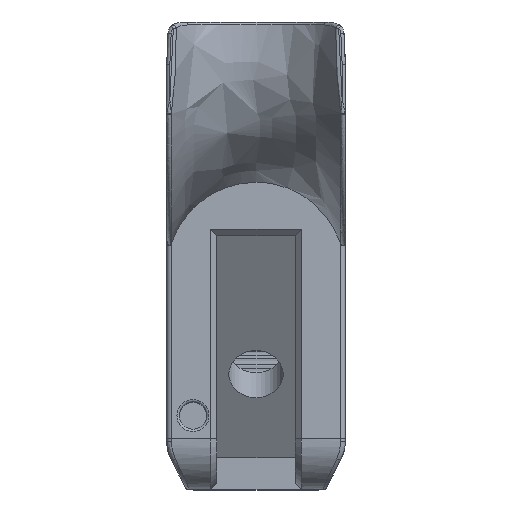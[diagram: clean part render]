
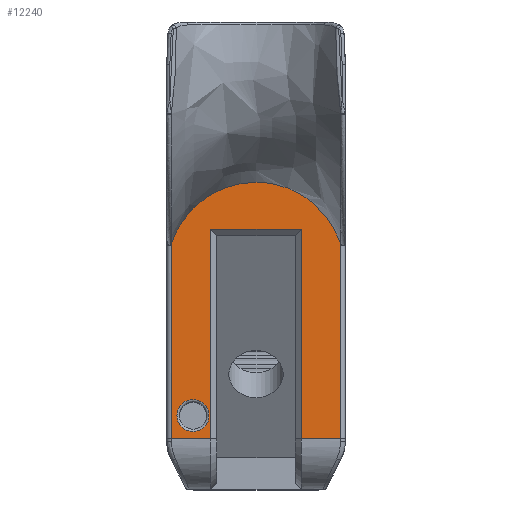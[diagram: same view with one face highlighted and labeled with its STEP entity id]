
A CAD part, top view. The second image highlights one B-rep face of the part: STEP entity #12240.
In plain terms, the highlighted planar face has unit normal (0, 0, 1).
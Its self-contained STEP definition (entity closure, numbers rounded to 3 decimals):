
#243=FACE_BOUND('',#2717,.T.);
#280=PLANE('',#13243);
#452=LINE('',#20827,#1044);
#459=LINE('',#20843,#1051);
#461=LINE('',#21357,#1053);
#485=LINE('',#22272,#1077);
#486=LINE('',#22274,#1078);
#487=LINE('',#22276,#1079);
#488=LINE('',#22278,#1080);
#1044=VECTOR('',#14233,10.);
#1051=VECTOR('',#14250,10.);
#1053=VECTOR('',#14288,10.);
#1077=VECTOR('',#14618,10.);
#1078=VECTOR('',#14619,10.);
#1079=VECTOR('',#14620,10.);
#1080=VECTOR('',#14621,10.);
#1942=FACE_OUTER_BOUND('',#2716,.T.);
#2716=EDGE_LOOP('',(#8739,#8740,#8741,#8742,#8743,#8744,#8745,#8746,#8747));
#2717=EDGE_LOOP('',(#8748));
#3450=B_SPLINE_CURVE_WITH_KNOTS('',3,(#22280,#22281,#22282,#22283,#22284,
#22285,#22286,#22287,#22288,#22289),.UNSPECIFIED.,.F.,.F.,(4,2,2,2,4),(0.313,
0.444,0.89,1.331,1.71),
 .UNSPECIFIED.);
#3451=B_SPLINE_CURVE_WITH_KNOTS('',3,(#22290,#22291,#22292,#22293,#22294,
#22295,#22296,#22297,#22298,#22299,#22300,#22301),.UNSPECIFIED.,.F.,.F.,
(4,2,2,2,2,4),(1.71,1.762,2.19,2.624,
3.022,3.107),.UNSPECIFIED.);
#4323=CIRCLE('',#13095,2.);
#4804=VERTEX_POINT('',#20825);
#4805=VERTEX_POINT('',#20826);
#4809=VERTEX_POINT('',#20842);
#4825=VERTEX_POINT('',#21356);
#4828=VERTEX_POINT('',#21369);
#4902=VERTEX_POINT('',#22271);
#4903=VERTEX_POINT('',#22273);
#4904=VERTEX_POINT('',#22275);
#4905=VERTEX_POINT('',#22277);
#4906=VERTEX_POINT('',#22279);
#6153=EDGE_CURVE('',#4804,#4805,#452,.T.);
#6162=EDGE_CURVE('',#4809,#4805,#459,.T.);
#6193=EDGE_CURVE('',#4809,#4825,#461,.T.);
#6198=EDGE_CURVE('',#4828,#4828,#4323,.T.);
#6338=EDGE_CURVE('',#4902,#4804,#485,.T.);
#6339=EDGE_CURVE('',#4903,#4902,#486,.T.);
#6340=EDGE_CURVE('',#4904,#4903,#487,.T.);
#6341=EDGE_CURVE('',#4905,#4904,#488,.T.);
#6342=EDGE_CURVE('',#4905,#4906,#3450,.T.);
#6343=EDGE_CURVE('',#4906,#4825,#3451,.T.);
#8739=ORIENTED_EDGE('',*,*,#6338,.F.);
#8740=ORIENTED_EDGE('',*,*,#6339,.F.);
#8741=ORIENTED_EDGE('',*,*,#6340,.F.);
#8742=ORIENTED_EDGE('',*,*,#6341,.F.);
#8743=ORIENTED_EDGE('',*,*,#6342,.T.);
#8744=ORIENTED_EDGE('',*,*,#6343,.T.);
#8745=ORIENTED_EDGE('',*,*,#6193,.F.);
#8746=ORIENTED_EDGE('',*,*,#6162,.T.);
#8747=ORIENTED_EDGE('',*,*,#6153,.F.);
#8748=ORIENTED_EDGE('',*,*,#6198,.F.);
#12240=ADVANCED_FACE('',(#1942,#243),#280,.T.);
#13095=AXIS2_PLACEMENT_3D('',#21370,#14298,#14299);
#13243=AXIS2_PLACEMENT_3D('',#22270,#14616,#14617);
#14233=DIRECTION('',(0.,-1.,0.));
#14250=DIRECTION('',(1.,0.,0.));
#14288=DIRECTION('',(0.,1.,0.));
#14298=DIRECTION('center_axis',(0.,0.,
1.));
#14299=DIRECTION('ref_axis',(1.,0.,0.));
#14616=DIRECTION('center_axis',(0.,0.,
1.));
#14617=DIRECTION('ref_axis',(0.,-1.,0.));
#14618=DIRECTION('',(-1.,0.,0.));
#14619=DIRECTION('',(0.,1.,0.));
#14620=DIRECTION('',(-1.,0.,0.));
#14621=DIRECTION('',(0.,-1.,0.));
#20825=CARTESIAN_POINT('',(18.417,-117.318,28.406));
#20826=CARTESIAN_POINT('',(18.417,-143.468,28.406));
#20827=CARTESIAN_POINT('',(18.417,-114.618,28.406));
#20842=CARTESIAN_POINT('',(13.518,-143.468,28.406));
#20843=CARTESIAN_POINT('',(28.956,-143.468,28.406));
#21356=CARTESIAN_POINT('',(13.518,-119.074,28.406));
#21357=CARTESIAN_POINT('',(13.518,-40.367,28.406));
#21369=CARTESIAN_POINT('',(18.205,-140.572,28.406));
#21370=CARTESIAN_POINT('Origin',(16.205,-140.572,28.406));
#22270=CARTESIAN_POINT('Origin',(19.207,-112.624,28.406));
#22271=CARTESIAN_POINT('',(29.746,-117.318,28.406));
#22272=CARTESIAN_POINT('',(24.173,-117.318,28.406));
#22273=CARTESIAN_POINT('',(29.746,-143.468,28.406));
#22274=CARTESIAN_POINT('',(29.746,-114.618,28.406));
#22275=CARTESIAN_POINT('',(34.645,-143.468,28.406));
#22276=CARTESIAN_POINT('',(19.207,-143.468,28.406));
#22277=CARTESIAN_POINT('',(34.645,-119.074,28.406));
#22278=CARTESIAN_POINT('',(34.645,-40.367,28.406));
#22279=CARTESIAN_POINT('',(24.081,-111.416,28.406));
#22280=CARTESIAN_POINT('Ctrl Pts',(34.645,-119.074,28.406));
#22281=CARTESIAN_POINT('Ctrl Pts',(34.504,-118.659,28.406));
#22282=CARTESIAN_POINT('Ctrl Pts',(34.339,-118.252,28.406));
#22283=CARTESIAN_POINT('Ctrl Pts',(33.514,-116.514,28.406));
#22284=CARTESIAN_POINT('Ctrl Pts',(32.621,-115.308,28.406));
#22285=CARTESIAN_POINT('Ctrl Pts',(30.434,-113.323,28.406));
#22286=CARTESIAN_POINT('Ctrl Pts',(29.164,-112.556,28.406));
#22287=CARTESIAN_POINT('Ctrl Pts',(26.592,-111.634,28.406));
#22288=CARTESIAN_POINT('Ctrl Pts',(25.341,-111.416,28.406));
#22289=CARTESIAN_POINT('Ctrl Pts',(24.081,-111.416,28.406));
#22290=CARTESIAN_POINT('Ctrl Pts',(24.081,-111.416,28.406));
#22291=CARTESIAN_POINT('Ctrl Pts',(23.907,-111.416,28.406));
#22292=CARTESIAN_POINT('Ctrl Pts',(23.733,-111.42,28.406));
#22293=CARTESIAN_POINT('Ctrl Pts',(22.136,-111.497,28.406));
#22294=CARTESIAN_POINT('Ctrl Pts',(20.743,-111.842,28.406));
#22295=CARTESIAN_POINT('Ctrl Pts',(18.138,-113.053,28.406));
#22296=CARTESIAN_POINT('Ctrl Pts',(16.956,-113.915,28.406));
#22297=CARTESIAN_POINT('Ctrl Pts',(15.066,-115.943,28.406));
#22298=CARTESIAN_POINT('Ctrl Pts',(14.34,-117.063,28.406));
#22299=CARTESIAN_POINT('Ctrl Pts',(13.71,-118.541,28.406));
#22300=CARTESIAN_POINT('Ctrl Pts',(13.609,-118.806,28.406));
#22301=CARTESIAN_POINT('Ctrl Pts',(13.518,-119.074,28.406));
